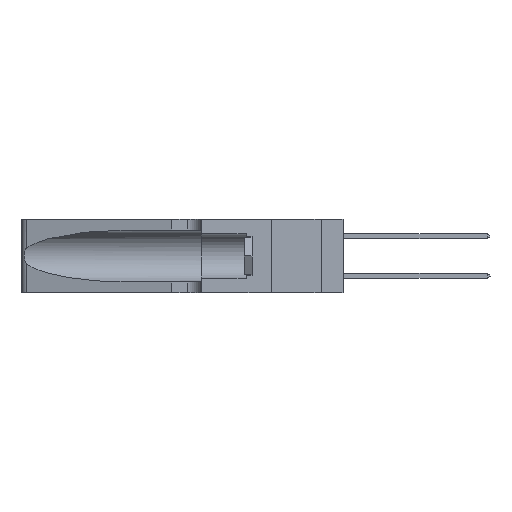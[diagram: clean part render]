
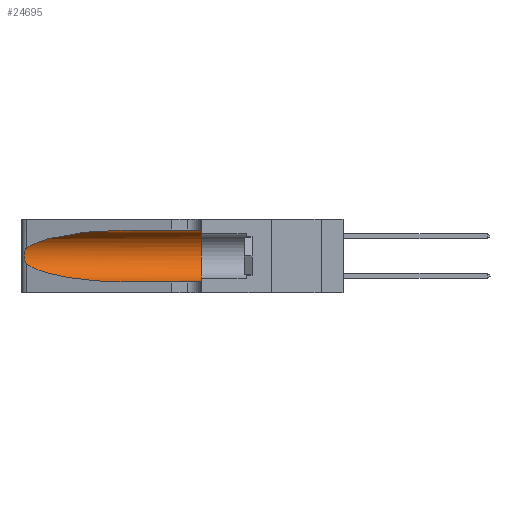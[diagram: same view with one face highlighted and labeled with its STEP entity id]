
A CAD part, left-side view. The second image highlights one B-rep face of the part: STEP entity #24695.
In plain terms, the highlighted cylindrical face has radius 3.308 mm (diameter 6.617 mm), a partial arc.
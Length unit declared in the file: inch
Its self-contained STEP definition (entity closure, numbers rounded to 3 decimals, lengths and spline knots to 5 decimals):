
#591 = CARTESIAN_POINT ( 'NONE',  ( 0.25487, 1.22718, 0.22369 ) ) ;
#750 = CARTESIAN_POINT ( 'NONE',  ( 0.26075, 1.23896, 0.178 ) ) ;
#1118 = CARTESIAN_POINT ( 'NONE',  ( 0.25487, 1.22718, 0.22369 ) ) ;
#1204 = EDGE_CURVE ( 'NONE', #41906, #6957, #45751, .T. ) ;
#1338 = EDGE_CURVE ( 'NONE', #9192, #41906, #30257, .T. ) ;
#1789 = CARTESIAN_POINT ( 'NONE',  ( 0.1305, 1.61858, 0.31525 ) ) ;
#3434 = CARTESIAN_POINT ( 'NONE',  ( 0.18966, 0.96281, 0.05475 ) ) ;
#4486 = CARTESIAN_POINT ( 'NONE',  ( 0.25856, 1.23593, 0.16098 ) ) ;
#6003 = CARTESIAN_POINT ( 'NONE',  ( 0.1305, 0.35, 0.05475 ) ) ;
#6957 = VERTEX_POINT ( 'NONE', #6003 ) ;
#8172 = VERTEX_POINT ( 'NONE', #42090 ) ;
#8189 = CARTESIAN_POINT ( 'NONE',  ( 0.25639, 1.23186, 0.15144 ) ) ;
#9192 = VERTEX_POINT ( 'NONE', #24245 ) ;
#10736 = CARTESIAN_POINT ( 'NONE',  ( 0.2373, 1.15595, 0.08982 ) ) ;
#11925 = CARTESIAN_POINT ( 'NONE',  ( 0.25487, 1.22718, 0.14631 ) ) ;
#15468 = CARTESIAN_POINT ( 'NONE',  ( 0.25639, 1.23184, 0.21858 ) ) ;
#15552 = CARTESIAN_POINT ( 'NONE',  ( 0.1305, 0.35, 0.31525 ) ) ;
#15817 = CARTESIAN_POINT ( 'NONE',  ( 0.18966, 0.96281, 0.31525 ) ) ;
#15859 = DIRECTION ( 'NONE',  ( 0., 1., 0. ) ) ;
#17085 = DIRECTION ( 'NONE',  ( 0., -1., 0. ) ) ;
#17517 = DIRECTION ( 'NONE',  ( 0., -1., 0. ) ) ;
#17891 = LINE ( 'NONE', #39519, #38594 ) ;
#18111 = CARTESIAN_POINT ( 'NONE',  ( 0.25487, 1.22718, 0.14631 ) ) ;
#18879 = EDGE_CURVE ( 'NONE', #8172, #6957, #17891, .T. ) ;
#19150 = CARTESIAN_POINT ( 'NONE',  ( 0.25854, 1.2359, 0.20912 ) ) ;
#19625 = ORIENTED_EDGE ( 'NONE', *, *, #18879, .T. ) ;
#20494 = VECTOR ( 'NONE', #38489, 39.37008 ) ;
#22102 = ORIENTED_EDGE ( 'NONE', *, *, #23753, .T. ) ;
#22707 = CARTESIAN_POINT ( 'NONE',  ( 0.25555, 1.22994, 0.2215 ) ) ;
#22870 = CARTESIAN_POINT ( 'NONE',  ( 0.26075, 1.23896, 0.19203 ) ) ;
#23213 = CARTESIAN_POINT ( 'NONE',  ( 0.2373, 1.15595, 0.28018 ) ) ;
#23242 = VERTEX_POINT ( 'NONE', #35150 ) ;
#23753 = EDGE_CURVE ( 'NONE', #9192, #23242, #37923, .T. ) ;
#24245 = CARTESIAN_POINT ( 'NONE',  ( 0.1305, 0.72297, 0.31525 ) ) ;
#24502 = CARTESIAN_POINT ( 'NONE',  ( 0.1305, 1.61858, 0.185 ) ) ;
#24695 = ADVANCED_FACE ( 'NONE', ( #34097 ), #32962, .F. ) ;
#26551 = CARTESIAN_POINT ( 'NONE',  ( 0.26017, 1.23833, 0.17102 ) ) ;
#26878 = EDGE_CURVE ( 'NONE', #23242, #36199, #29393, .T. ) ;
#28759 = CARTESIAN_POINT ( 'NONE',  ( 0.25487, 1.22718, 0.14631 ) ) ;
#29232 = CARTESIAN_POINT ( 'NONE',  ( 0.1305, 0.72297, 0.05475 ) ) ;
#29393 = B_SPLINE_CURVE_WITH_KNOTS ( 'NONE', 3,
 ( #591, #22707, #15468, #41162, #19150, #44832, #22870, #750, #26551, #4486, #30250, #8189, #33960, #11925 ),
 .UNSPECIFIED., .F., .F.,
 ( 4, 2, 2, 2, 2, 2, 4 ),
 ( 0., 0.00027, 0.00053, 0.00107, 0.0016, 0.00187, 0.00214 ),
 .UNSPECIFIED. ) ;
#30250 = CARTESIAN_POINT ( 'NONE',  ( 0.25789, 1.23486, 0.15765 ) ) ;
#30257 = LINE ( 'NONE', #1789, #20494 ) ;
#30824 = EDGE_CURVE ( 'NONE', #36199, #8172, #42889, .T. ) ;
#32249 = ORIENTED_EDGE ( 'NONE', *, *, #30824, .T. ) ;
#32962 = CYLINDRICAL_SURFACE ( 'NONE', #43982, 0.13025 ) ;
#33960 = CARTESIAN_POINT ( 'NONE',  ( 0.25555, 1.22993, 0.14849 ) ) ;
#34097 = FACE_OUTER_BOUND ( 'NONE', #35695, .T. ) ;
#35150 = CARTESIAN_POINT ( 'NONE',  ( 0.25487, 1.22718, 0.22369 ) ) ;
#35695 = EDGE_LOOP ( 'NONE', ( #22102, #42545, #32249, #19625, #45233, #42380 ) ) ;
#36199 = VERTEX_POINT ( 'NONE', #28759 ) ;
#37875 = CARTESIAN_POINT ( 'NONE',  ( 0.1305, 0.35, 0.185 ) ) ;
#37923 =( BOUNDED_CURVE ( )  B_SPLINE_CURVE ( 3, ( #41499, #15817, #23213, #1118 ),
 .UNSPECIFIED., .F., .F. ) 
 B_SPLINE_CURVE_WITH_KNOTS ( ( 4, 4 ),
 ( 1.5708, 2.84003 ),
 .UNSPECIFIED. ) 
 CURVE ( )  GEOMETRIC_REPRESENTATION_ITEM ( )  RATIONAL_B_SPLINE_CURVE ( ( 1., 0.87, 0.87, 1. ) ) 
 REPRESENTATION_ITEM ( '' )  );
#38489 = DIRECTION ( 'NONE',  ( 0., -1., 0. ) ) ;
#38594 = VECTOR ( 'NONE', #17517, 39.37008 ) ;
#39519 = CARTESIAN_POINT ( 'NONE',  ( 0.1305, 1.61858, 0.05475 ) ) ;
#41113 = AXIS2_PLACEMENT_3D ( 'NONE', #37875, #15859, #41539 ) ;
#41162 = CARTESIAN_POINT ( 'NONE',  ( 0.25787, 1.23484, 0.2124 ) ) ;
#41499 = CARTESIAN_POINT ( 'NONE',  ( 0.1305, 0.72297, 0.31525 ) ) ;
#41539 = DIRECTION ( 'NONE',  ( 0., 0., 1. ) ) ;
#41906 = VERTEX_POINT ( 'NONE', #15552 ) ;
#42090 = CARTESIAN_POINT ( 'NONE',  ( 0.1305, 0.72297, 0.05475 ) ) ;
#42380 = ORIENTED_EDGE ( 'NONE', *, *, #1338, .F. ) ;
#42545 = ORIENTED_EDGE ( 'NONE', *, *, #26878, .T. ) ;
#42769 = DIRECTION ( 'NONE',  ( 0., 0., -1. ) ) ;
#42889 =( BOUNDED_CURVE ( )  B_SPLINE_CURVE ( 3, ( #18111, #10736, #3434, #29232 ),
 .UNSPECIFIED., .F., .F. ) 
 B_SPLINE_CURVE_WITH_KNOTS ( ( 4, 4 ),
 ( 3.44316, 4.71239 ),
 .UNSPECIFIED. ) 
 CURVE ( )  GEOMETRIC_REPRESENTATION_ITEM ( )  RATIONAL_B_SPLINE_CURVE ( ( 1., 0.87, 0.87, 1. ) ) 
 REPRESENTATION_ITEM ( '' )  );
#43982 = AXIS2_PLACEMENT_3D ( 'NONE', #24502, #17085, #42769 ) ;
#44832 = CARTESIAN_POINT ( 'NONE',  ( 0.26018, 1.23835, 0.19895 ) ) ;
#45233 = ORIENTED_EDGE ( 'NONE', *, *, #1204, .F. ) ;
#45751 = CIRCLE ( 'NONE', #41113, 0.13025 ) ;
